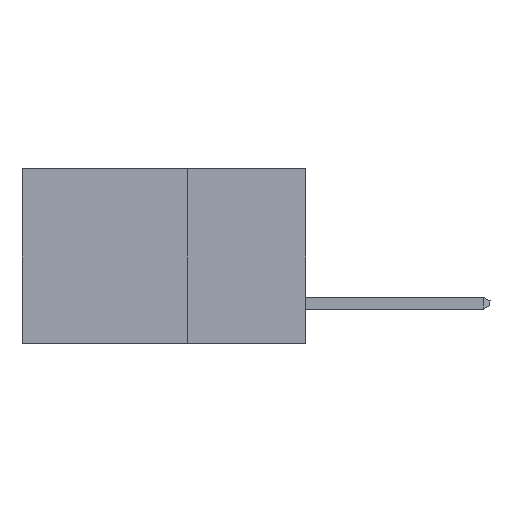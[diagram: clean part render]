
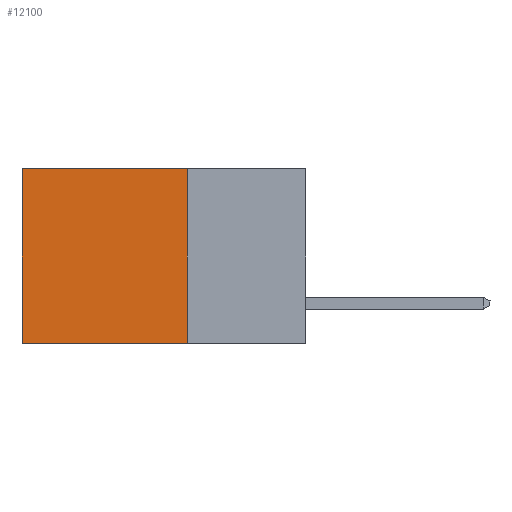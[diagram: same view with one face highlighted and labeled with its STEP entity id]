
A CAD part, left-side view. The second image highlights one B-rep face of the part: STEP entity #12100.
In plain terms, the highlighted planar face has unit normal (-1, 0, 0).
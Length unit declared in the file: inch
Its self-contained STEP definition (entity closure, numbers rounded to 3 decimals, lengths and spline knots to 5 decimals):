
#46 = EDGE_CURVE ( 'NONE', #4606, #4958, #10529, .T. ) ;
#711 = VECTOR ( 'NONE', #8356, 39.37008 ) ;
#1294 = CARTESIAN_POINT ( 'NONE',  ( 0.2615, 0.25, 0. ) ) ;
#3023 = FACE_OUTER_BOUND ( 'NONE', #12258, .T. ) ;
#3432 = VECTOR ( 'NONE', #11566, 39.37008 ) ;
#3636 = CARTESIAN_POINT ( 'NONE',  ( 0.2615, 0.25, -0.37 ) ) ;
#3818 = AXIS2_PLACEMENT_3D ( 'NONE', #10954, #9907, #13231 ) ;
#4606 = VERTEX_POINT ( 'NONE', #5991 ) ;
#4759 = CARTESIAN_POINT ( 'NONE',  ( 0.2615, 0.6, -0.37 ) ) ;
#4958 = VERTEX_POINT ( 'NONE', #12250 ) ;
#5020 = CARTESIAN_POINT ( 'NONE',  ( 0.2615, 0.25, -0.37 ) ) ;
#5115 = LINE ( 'NONE', #9563, #12785 ) ;
#5400 = PLANE ( 'NONE',  #3818 ) ;
#5991 = CARTESIAN_POINT ( 'NONE',  ( 0.2615, 0.6, 0. ) ) ;
#6308 = ORIENTED_EDGE ( 'NONE', *, *, #6912, .F. ) ;
#6912 = EDGE_CURVE ( 'NONE', #12425, #11322, #11999, .T. ) ;
#7209 = CARTESIAN_POINT ( 'NONE',  ( 0.2615, 0.25, -0.37 ) ) ;
#8356 = DIRECTION ( 'NONE',  ( 0., 1., 0. ) ) ;
#8559 = EDGE_CURVE ( 'NONE', #11322, #4958, #9248, .T. ) ;
#8971 = VECTOR ( 'NONE', #9583, 39.37008 ) ;
#9248 = LINE ( 'NONE', #5020, #711 ) ;
#9550 = ORIENTED_EDGE ( 'NONE', *, *, #11427, .T. ) ;
#9563 = CARTESIAN_POINT ( 'NONE',  ( 0.2615, 0.25, 0. ) ) ;
#9583 = DIRECTION ( 'NONE',  ( 0., 0., -1. ) ) ;
#9633 = DIRECTION ( 'NONE',  ( 0., 1., 0. ) ) ;
#9907 = DIRECTION ( 'NONE',  ( 1., 0., 0. ) ) ;
#10529 = LINE ( 'NONE', #4759, #3432 ) ;
#10954 = CARTESIAN_POINT ( 'NONE',  ( 0.2615, 0.25, -0.37 ) ) ;
#11322 = VERTEX_POINT ( 'NONE', #3636 ) ;
#11427 = EDGE_CURVE ( 'NONE', #12425, #4606, #5115, .T. ) ;
#11566 = DIRECTION ( 'NONE',  ( 0., 0., -1. ) ) ;
#11930 = ORIENTED_EDGE ( 'NONE', *, *, #46, .T. ) ;
#11999 = LINE ( 'NONE', #7209, #8971 ) ;
#12100 = ADVANCED_FACE ( 'NONE', ( #3023 ), #5400, .F. ) ;
#12250 = CARTESIAN_POINT ( 'NONE',  ( 0.2615, 0.6, -0.37 ) ) ;
#12258 = EDGE_LOOP ( 'NONE', ( #11930, #12715, #6308, #9550 ) ) ;
#12425 = VERTEX_POINT ( 'NONE', #1294 ) ;
#12715 = ORIENTED_EDGE ( 'NONE', *, *, #8559, .F. ) ;
#12785 = VECTOR ( 'NONE', #9633, 39.37008 ) ;
#13231 = DIRECTION ( 'NONE',  ( 0., 0., -1. ) ) ;
